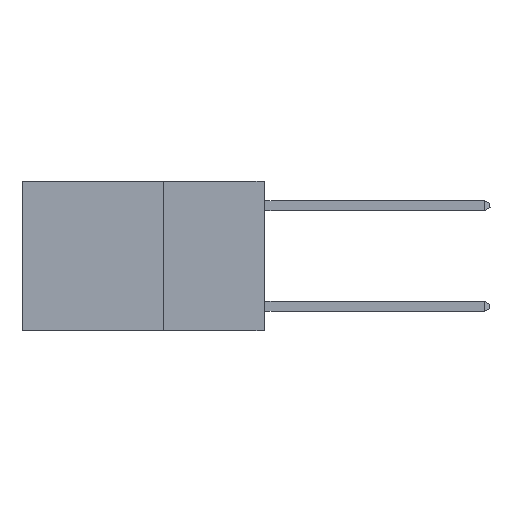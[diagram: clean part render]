
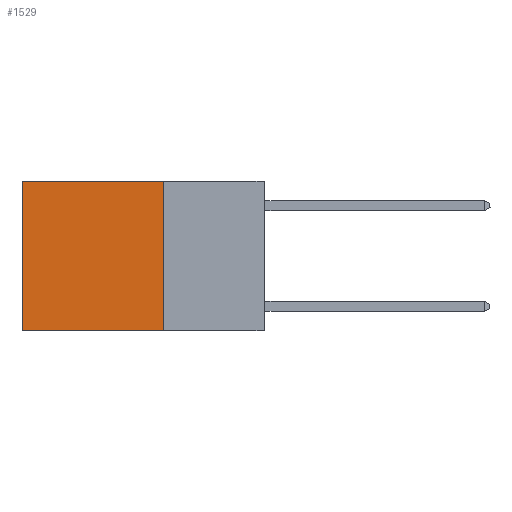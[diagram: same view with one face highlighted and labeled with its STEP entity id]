
A CAD part, left-side view. The second image highlights one B-rep face of the part: STEP entity #1529.
In plain terms, the highlighted planar face has unit normal (-1, 0, 0).
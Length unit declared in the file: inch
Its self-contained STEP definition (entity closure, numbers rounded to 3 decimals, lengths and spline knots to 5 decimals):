
#28 = DIRECTION ( 'NONE',  ( 0., 1., 0. ) ) ;
#1278 = PLANE ( 'NONE',  #1798 ) ;
#1529 = ADVANCED_FACE ( 'NONE', ( #8711 ), #1278, .F. ) ;
#1798 = AXIS2_PLACEMENT_3D ( 'NONE', #15277, #5956, #13905 ) ;
#2696 = ORIENTED_EDGE ( 'NONE', *, *, #11578, .T. ) ;
#3500 = EDGE_CURVE ( 'NONE', #16231, #11060, #17960, .T. ) ;
#4044 = CARTESIAN_POINT ( 'NONE',  ( 0.2625, 0.6, -0.37 ) ) ;
#4111 = LINE ( 'NONE', #13215, #11928 ) ;
#5221 = DIRECTION ( 'NONE',  ( 0., 0., -1. ) ) ;
#5255 = VECTOR ( 'NONE', #13833, 39.37008 ) ;
#5602 = DIRECTION ( 'NONE',  ( 0., 0., -1. ) ) ;
#5947 = CARTESIAN_POINT ( 'NONE',  ( 0.2625, 0.25, 0. ) ) ;
#5956 = DIRECTION ( 'NONE',  ( 1., 0., 0. ) ) ;
#6170 = CARTESIAN_POINT ( 'NONE',  ( 0.2625, 0.25, -0.37 ) ) ;
#6309 = VERTEX_POINT ( 'NONE', #19447 ) ;
#6617 = LINE ( 'NONE', #6170, #13409 ) ;
#6777 = VECTOR ( 'NONE', #5221, 39.37008 ) ;
#8356 = CARTESIAN_POINT ( 'NONE',  ( 0.2625, 0.6, 0. ) ) ;
#8708 = EDGE_CURVE ( 'NONE', #11926, #6309, #4111, .T. ) ;
#8711 = FACE_OUTER_BOUND ( 'NONE', #10875, .T. ) ;
#9435 = LINE ( 'NONE', #5947, #5255 ) ;
#10875 = EDGE_LOOP ( 'NONE', ( #17937, #17962, #11706, #2696 ) ) ;
#11060 = VERTEX_POINT ( 'NONE', #4044 ) ;
#11578 = EDGE_CURVE ( 'NONE', #11926, #16231, #9435, .T. ) ;
#11706 = ORIENTED_EDGE ( 'NONE', *, *, #8708, .F. ) ;
#11926 = VERTEX_POINT ( 'NONE', #13664 ) ;
#11928 = VECTOR ( 'NONE', #5602, 39.37008 ) ;
#13215 = CARTESIAN_POINT ( 'NONE',  ( 0.2625, 0.25, 0. ) ) ;
#13409 = VECTOR ( 'NONE', #28, 39.37008 ) ;
#13664 = CARTESIAN_POINT ( 'NONE',  ( 0.2625, 0.25, 0. ) ) ;
#13833 = DIRECTION ( 'NONE',  ( 0., 1., 0. ) ) ;
#13905 = DIRECTION ( 'NONE',  ( 0., 0., -1. ) ) ;
#14608 = EDGE_CURVE ( 'NONE', #6309, #11060, #6617, .T. ) ;
#15277 = CARTESIAN_POINT ( 'NONE',  ( 0.2625, 0.25, 0. ) ) ;
#16049 = CARTESIAN_POINT ( 'NONE',  ( 0.2625, 0.6, 0. ) ) ;
#16231 = VERTEX_POINT ( 'NONE', #16049 ) ;
#17937 = ORIENTED_EDGE ( 'NONE', *, *, #3500, .T. ) ;
#17960 = LINE ( 'NONE', #8356, #6777 ) ;
#17962 = ORIENTED_EDGE ( 'NONE', *, *, #14608, .F. ) ;
#19447 = CARTESIAN_POINT ( 'NONE',  ( 0.2625, 0.25, -0.37 ) ) ;
